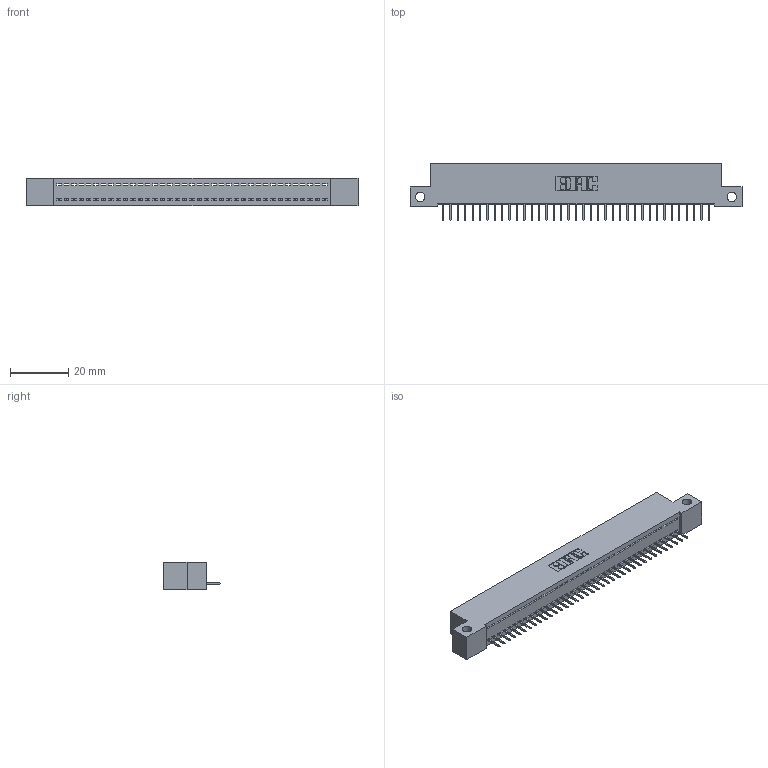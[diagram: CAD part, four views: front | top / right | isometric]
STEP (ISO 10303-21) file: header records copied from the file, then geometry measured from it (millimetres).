
FILE_DESCRIPTION (( 'STEP AP203' ), '1' );
FILE_NAME ('342-037-524-112.STEP', '2019-10-02T14:05:11', ( '' ), ( '' ), 'SwSTEP 2.0', 'SolidWorks 2016', '' );
FILE_SCHEMA (( 'CONFIG_CONTROL_DESIGN' ));
Length unit declared in the file: inch
Products named in the file (3): 342-037-524-112; 342 Part_Side Mount; 345-292-001_345-293-124
Assembly tree (38 placements, depth 2):
  342-037-524-112
    342 Part_Side Mount
    345-292-001_345-293-124  x37
Bounding box: 114.3 x 19.69 x 9.4 mm (x, y, z)
Volume: 9783.3 mm3; surface area: 13655.9 mm2
Topology: 38 solids, 38 shells, 2404 faces, 6959 edges, 4490 vertices
Faces by surface type: plane 1842, cylinder 562
Entity records: 23211 total; most frequent: CARTESIAN_POINT 4009, ORIENTED_EDGE 3982, DIRECTION 3393, EDGE_CURVE 1991, LINE 1867, VECTOR 1867, VERTEX_POINT 1322, AXIS2_PLACEMENT_3D 763
